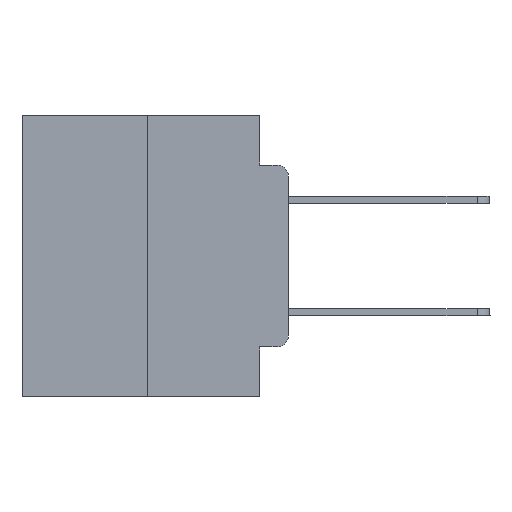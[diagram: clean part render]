
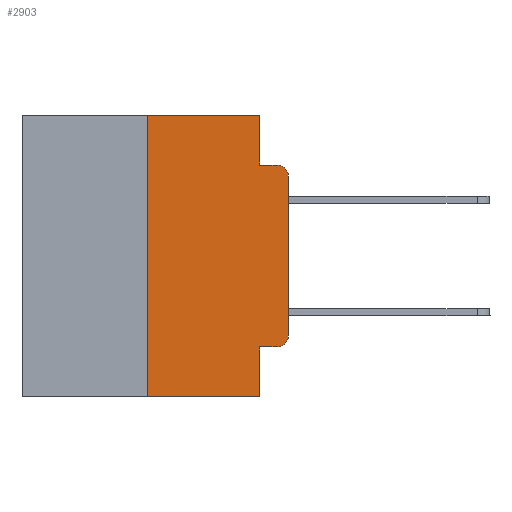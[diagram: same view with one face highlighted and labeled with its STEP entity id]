
A CAD part, left-side view. The second image highlights one B-rep face of the part: STEP entity #2903.
In plain terms, the highlighted planar face has unit normal (-1, 0, 0).
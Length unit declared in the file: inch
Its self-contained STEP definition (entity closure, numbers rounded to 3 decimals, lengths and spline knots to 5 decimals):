
#435 = AXIS2_PLACEMENT_3D ( 'NONE', #16757, #25335, #6051 ) ;
#857 = CARTESIAN_POINT ( 'NONE',  ( 0., 0.051, -0.0885 ) ) ;
#1481 = LINE ( 'NONE', #12592, #4839 ) ;
#1679 = ORIENTED_EDGE ( 'NONE', *, *, #7891, .T. ) ;
#1697 = CARTESIAN_POINT ( 'NONE',  ( 0., 0.02, -0.0885 ) ) ;
#1905 = VECTOR ( 'NONE', #27599, 39.37008 ) ;
#2010 = LINE ( 'NONE', #6229, #24844 ) ;
#2360 = EDGE_CURVE ( 'NONE', #21215, #9094, #27320, .T. ) ;
#2842 = LINE ( 'NONE', #7189, #17486 ) ;
#2903 = ADVANCED_FACE ( 'NONE', ( #8431 ), #8159, .F. ) ;
#3248 = VERTEX_POINT ( 'NONE', #27106 ) ;
#3331 = ORIENTED_EDGE ( 'NONE', *, *, #2360, .F. ) ;
#3639 = EDGE_CURVE ( 'NONE', #16089, #14852, #2010, .T. ) ;
#3870 = CARTESIAN_POINT ( 'NONE',  ( 0., 0., -0.3915 ) ) ;
#4549 = VERTEX_POINT ( 'NONE', #8960 ) ;
#4839 = VECTOR ( 'NONE', #27205, 39.37008 ) ;
#5318 = EDGE_LOOP ( 'NONE', ( #15284, #16170, #15629, #3331, #11259, #5591, #1679, #8098, #9965, #25823 ) ) ;
#5324 = EDGE_CURVE ( 'NONE', #9094, #20873, #14725, .T. ) ;
#5591 = ORIENTED_EDGE ( 'NONE', *, *, #3639, .F. ) ;
#5617 = DIRECTION ( 'NONE',  ( -1., 0., 0. ) ) ;
#6051 = DIRECTION ( 'NONE',  ( 0., 0., -1. ) ) ;
#6229 = CARTESIAN_POINT ( 'NONE',  ( 0., 0.25, 0. ) ) ;
#6405 = CIRCLE ( 'NONE', #16742, 0.02 ) ;
#7040 = VECTOR ( 'NONE', #10077, 39.37008 ) ;
#7189 = CARTESIAN_POINT ( 'NONE',  ( 0., 0.051, 0. ) ) ;
#7401 = VERTEX_POINT ( 'NONE', #10285 ) ;
#7744 = AXIS2_PLACEMENT_3D ( 'NONE', #9559, #9974, #14073 ) ;
#7891 = EDGE_CURVE ( 'NONE', #16089, #4549, #19080, .T. ) ;
#7952 = CARTESIAN_POINT ( 'NONE',  ( 0., 0.051, 0. ) ) ;
#8098 = ORIENTED_EDGE ( 'NONE', *, *, #20656, .F. ) ;
#8159 = PLANE ( 'NONE',  #435 ) ;
#8282 = VECTOR ( 'NONE', #16564, 39.37008 ) ;
#8324 = EDGE_CURVE ( 'NONE', #7401, #22054, #1481, .T. ) ;
#8431 = FACE_OUTER_BOUND ( 'NONE', #5318, .T. ) ;
#8652 = CARTESIAN_POINT ( 'NONE',  ( 0., 0.02, -0.4115 ) ) ;
#8960 = CARTESIAN_POINT ( 'NONE',  ( 0., 0.051, -0.5 ) ) ;
#9094 = VERTEX_POINT ( 'NONE', #857 ) ;
#9559 = CARTESIAN_POINT ( 'NONE',  ( 0., 0.02, -0.3915 ) ) ;
#9965 = ORIENTED_EDGE ( 'NONE', *, *, #8324, .T. ) ;
#9974 = DIRECTION ( 'NONE',  ( -1., 0., 0. ) ) ;
#10077 = DIRECTION ( 'NONE',  ( 0., -1., 0. ) ) ;
#10285 = CARTESIAN_POINT ( 'NONE',  ( 0., 0.051, -0.4115 ) ) ;
#10444 = DIRECTION ( 'NONE',  ( 0., 0., 1. ) ) ;
#10578 = CARTESIAN_POINT ( 'NONE',  ( 0., 0.473, 0. ) ) ;
#10726 = LINE ( 'NONE', #10578, #20223 ) ;
#11259 = ORIENTED_EDGE ( 'NONE', *, *, #12462, .F. ) ;
#12462 = EDGE_CURVE ( 'NONE', #14852, #21215, #10726, .T. ) ;
#12592 = CARTESIAN_POINT ( 'NONE',  ( 0., 0.051, -0.4115 ) ) ;
#14044 = CIRCLE ( 'NONE', #7744, 0.02 ) ;
#14073 = DIRECTION ( 'NONE',  ( 0., 0., -1. ) ) ;
#14305 = DIRECTION ( 'NONE',  ( 0., 0., 1. ) ) ;
#14725 = LINE ( 'NONE', #21061, #8282 ) ;
#14852 = VERTEX_POINT ( 'NONE', #19219 ) ;
#15284 = ORIENTED_EDGE ( 'NONE', *, *, #21905, .T. ) ;
#15629 = ORIENTED_EDGE ( 'NONE', *, *, #5324, .F. ) ;
#16089 = VERTEX_POINT ( 'NONE', #18292 ) ;
#16170 = ORIENTED_EDGE ( 'NONE', *, *, #25597, .T. ) ;
#16564 = DIRECTION ( 'NONE',  ( 0., -1., 0. ) ) ;
#16742 = AXIS2_PLACEMENT_3D ( 'NONE', #26712, #5617, #26854 ) ;
#16757 = CARTESIAN_POINT ( 'NONE',  ( 0., 0.473, 0. ) ) ;
#17476 = DIRECTION ( 'NONE',  ( 0., 0., -1. ) ) ;
#17486 = VECTOR ( 'NONE', #17476, 39.37008 ) ;
#18292 = CARTESIAN_POINT ( 'NONE',  ( 0., 0.25, -0.5 ) ) ;
#19080 = LINE ( 'NONE', #22907, #7040 ) ;
#19219 = CARTESIAN_POINT ( 'NONE',  ( 0., 0.25, 0. ) ) ;
#19315 = DIRECTION ( 'NONE',  ( 0., -1., 0. ) ) ;
#20223 = VECTOR ( 'NONE', #19315, 39.37008 ) ;
#20608 = VECTOR ( 'NONE', #14305, 39.37008 ) ;
#20656 = EDGE_CURVE ( 'NONE', #7401, #4549, #2842, .T. ) ;
#20873 = VERTEX_POINT ( 'NONE', #1697 ) ;
#21061 = CARTESIAN_POINT ( 'NONE',  ( 0., 0.051, -0.0885 ) ) ;
#21215 = VERTEX_POINT ( 'NONE', #7952 ) ;
#21254 = VERTEX_POINT ( 'NONE', #3870 ) ;
#21905 = EDGE_CURVE ( 'NONE', #21254, #3248, #22338, .T. ) ;
#22054 = VERTEX_POINT ( 'NONE', #8652 ) ;
#22338 = LINE ( 'NONE', #25142, #20608 ) ;
#22907 = CARTESIAN_POINT ( 'NONE',  ( 0., 0.473, -0.5 ) ) ;
#22990 = CARTESIAN_POINT ( 'NONE',  ( 0., 0.051, 0. ) ) ;
#24844 = VECTOR ( 'NONE', #10444, 39.37008 ) ;
#25142 = CARTESIAN_POINT ( 'NONE',  ( 0., 0., 0. ) ) ;
#25335 = DIRECTION ( 'NONE',  ( 1., 0., 0. ) ) ;
#25580 = EDGE_CURVE ( 'NONE', #22054, #21254, #14044, .T. ) ;
#25597 = EDGE_CURVE ( 'NONE', #3248, #20873, #6405, .T. ) ;
#25823 = ORIENTED_EDGE ( 'NONE', *, *, #25580, .T. ) ;
#26712 = CARTESIAN_POINT ( 'NONE',  ( 0., 0.02, -0.1085 ) ) ;
#26854 = DIRECTION ( 'NONE',  ( 0., 0., -1. ) ) ;
#27106 = CARTESIAN_POINT ( 'NONE',  ( 0., 0., -0.1085 ) ) ;
#27205 = DIRECTION ( 'NONE',  ( 0., -1., 0. ) ) ;
#27320 = LINE ( 'NONE', #22990, #1905 ) ;
#27599 = DIRECTION ( 'NONE',  ( 0., 0., -1. ) ) ;
